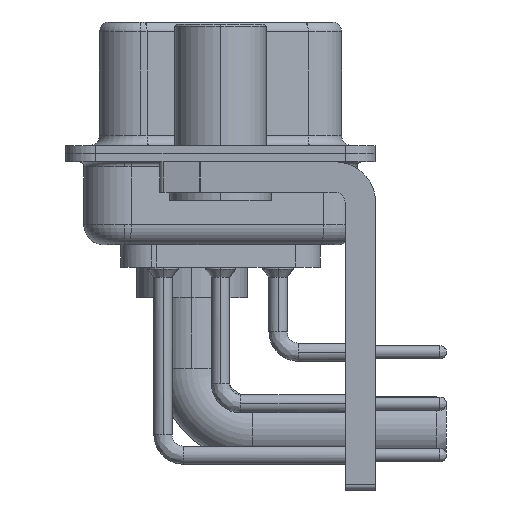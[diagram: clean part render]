
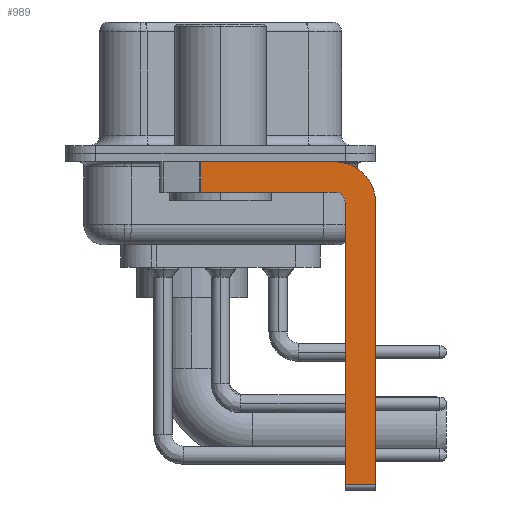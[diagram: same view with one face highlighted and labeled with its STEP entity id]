
A CAD part, left-side view. The second image highlights one B-rep face of the part: STEP entity #989.
In plain terms, the highlighted planar face has unit normal (-1, 0, 0).
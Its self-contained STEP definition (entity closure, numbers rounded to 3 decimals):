
#283 = EDGE_CURVE ( 'NONE', #38942, #8479, #36353, .T. ) ;
#812 = DIRECTION ( 'NONE',  ( 1., 0., 0. ) ) ;
#989 = ADVANCED_FACE ( 'NONE', ( #34324 ), #37566, .F. ) ;
#2116 = CARTESIAN_POINT ( 'NONE',  ( -2.9, -7.65, -2.4 ) ) ;
#3274 = CARTESIAN_POINT ( 'NONE',  ( -2.9, -5.65, -2.4 ) ) ;
#4101 = ORIENTED_EDGE ( 'NONE', *, *, #30331, .F. ) ;
#4162 = CARTESIAN_POINT ( 'NONE',  ( -2.9, -5.65, -16.35 ) ) ;
#4362 = LINE ( 'NONE', #4162, #18183 ) ;
#5792 = EDGE_CURVE ( 'NONE', #32294, #26912, #6336, .T. ) ;
#6336 = LINE ( 'NONE', #30591, #37295 ) ;
#8254 = VERTEX_POINT ( 'NONE', #26123 ) ;
#8479 = VERTEX_POINT ( 'NONE', #2116 ) ;
#8724 = AXIS2_PLACEMENT_3D ( 'NONE', #25613, #31294, #16349 ) ;
#8937 = DIRECTION ( 'NONE',  ( 1., 0., 0. ) ) ;
#9714 = ORIENTED_EDGE ( 'NONE', *, *, #19456, .F. ) ;
#9896 = CARTESIAN_POINT ( 'NONE',  ( -2.9, -5.65, -2.4 ) ) ;
#10764 = CARTESIAN_POINT ( 'NONE',  ( -2.9, -5.65, -0.4 ) ) ;
#10909 = DIRECTION ( 'NONE',  ( 0., 0., -1. ) ) ;
#11184 = AXIS2_PLACEMENT_3D ( 'NONE', #9896, #812, #31702 ) ;
#11198 = ORIENTED_EDGE ( 'NONE', *, *, #283, .F. ) ;
#11298 = ORIENTED_EDGE ( 'NONE', *, *, #32886, .T. ) ;
#11525 = LINE ( 'NONE', #33127, #15732 ) ;
#11768 = EDGE_CURVE ( 'NONE', #23464, #26912, #16966, .T. ) ;
#12204 = VECTOR ( 'NONE', #36805, 1000. ) ;
#12547 = EDGE_LOOP ( 'NONE', ( #9714, #17793, #15970, #31592, #28525, #11298, #4101, #11198 ) ) ;
#13934 = CARTESIAN_POINT ( 'NONE',  ( -2.9, 0.978, -1.9 ) ) ;
#15714 = AXIS2_PLACEMENT_3D ( 'NONE', #3274, #8937, #18605 ) ;
#15732 = VECTOR ( 'NONE', #23824, 1000. ) ;
#15970 = ORIENTED_EDGE ( 'NONE', *, *, #5792, .F. ) ;
#16056 = CARTESIAN_POINT ( 'NONE',  ( -2.9, 0.978, -0.4 ) ) ;
#16349 = DIRECTION ( 'NONE',  ( 0., 0., 1. ) ) ;
#16966 = LINE ( 'NONE', #13934, #36796 ) ;
#16968 = CARTESIAN_POINT ( 'NONE',  ( -2.9, -7.65, -16.35 ) ) ;
#17558 = VERTEX_POINT ( 'NONE', #16968 ) ;
#17793 = ORIENTED_EDGE ( 'NONE', *, *, #11768, .T. ) ;
#18183 = VECTOR ( 'NONE', #19308, 1000. ) ;
#18605 = DIRECTION ( 'NONE',  ( 0., 0., -1. ) ) ;
#18851 = DIRECTION ( 'NONE',  ( 0., 1., 0. ) ) ;
#19020 = CIRCLE ( 'NONE', #8724, 0.5 ) ;
#19308 = DIRECTION ( 'NONE',  ( 0., -1., 0. ) ) ;
#19456 = EDGE_CURVE ( 'NONE', #23464, #38942, #11525, .T. ) ;
#20954 = EDGE_CURVE ( 'NONE', #36535, #32294, #19020, .T. ) ;
#23464 = VERTEX_POINT ( 'NONE', #16056 ) ;
#23824 = DIRECTION ( 'NONE',  ( 0., -1., 0. ) ) ;
#24678 = LINE ( 'NONE', #33771, #12204 ) ;
#25024 = CARTESIAN_POINT ( 'NONE',  ( -2.9, -5.65, -1.9 ) ) ;
#25613 = CARTESIAN_POINT ( 'NONE',  ( -2.9, -5.65, -2.4 ) ) ;
#26123 = CARTESIAN_POINT ( 'NONE',  ( -2.9, -6.15, -16.35 ) ) ;
#26912 = VERTEX_POINT ( 'NONE', #27604 ) ;
#27326 = CARTESIAN_POINT ( 'NONE',  ( -2.9, -6.15, -2.4 ) ) ;
#27604 = CARTESIAN_POINT ( 'NONE',  ( -2.9, 0.978, -1.9 ) ) ;
#27966 = EDGE_CURVE ( 'NONE', #8254, #36535, #30236, .T. ) ;
#28525 = ORIENTED_EDGE ( 'NONE', *, *, #27966, .F. ) ;
#29622 = CARTESIAN_POINT ( 'NONE',  ( -2.9, -6.15, -16.6 ) ) ;
#30236 = LINE ( 'NONE', #29622, #35345 ) ;
#30331 = EDGE_CURVE ( 'NONE', #8479, #17558, #24678, .T. ) ;
#30591 = CARTESIAN_POINT ( 'NONE',  ( -2.9, -5.65, -1.9 ) ) ;
#31294 = DIRECTION ( 'NONE',  ( -1., 0., 0. ) ) ;
#31592 = ORIENTED_EDGE ( 'NONE', *, *, #20954, .F. ) ;
#31702 = DIRECTION ( 'NONE',  ( 0., 0., -1. ) ) ;
#32294 = VERTEX_POINT ( 'NONE', #25024 ) ;
#32886 = EDGE_CURVE ( 'NONE', #8254, #17558, #4362, .T. ) ;
#33127 = CARTESIAN_POINT ( 'NONE',  ( -2.9, 3., -0.4 ) ) ;
#33771 = CARTESIAN_POINT ( 'NONE',  ( -2.9, -7.65, -2.4 ) ) ;
#34324 = FACE_OUTER_BOUND ( 'NONE', #12547, .T. ) ;
#35345 = VECTOR ( 'NONE', #39525, 1000. ) ;
#36353 = CIRCLE ( 'NONE', #15714, 2. ) ;
#36535 = VERTEX_POINT ( 'NONE', #27326 ) ;
#36796 = VECTOR ( 'NONE', #10909, 1000. ) ;
#36805 = DIRECTION ( 'NONE',  ( 0., 0., -1. ) ) ;
#37295 = VECTOR ( 'NONE', #18851, 1000. ) ;
#37566 = PLANE ( 'NONE',  #11184 ) ;
#38942 = VERTEX_POINT ( 'NONE', #10764 ) ;
#39525 = DIRECTION ( 'NONE',  ( 0., 0., 1. ) ) ;
